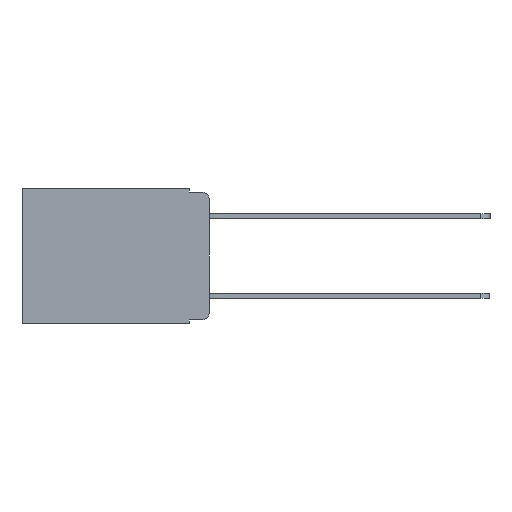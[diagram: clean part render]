
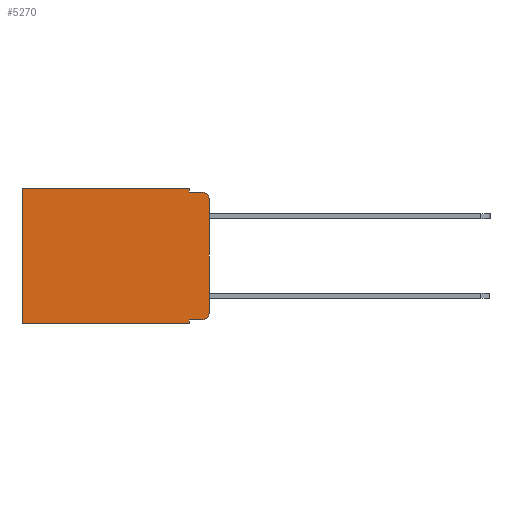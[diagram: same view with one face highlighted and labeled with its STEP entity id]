
A CAD part, left-side view. The second image highlights one B-rep face of the part: STEP entity #5270.
In plain terms, the highlighted planar face has unit normal (-1, 0, 0).
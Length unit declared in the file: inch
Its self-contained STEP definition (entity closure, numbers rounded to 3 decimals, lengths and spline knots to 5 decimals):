
#264 = AXIS2_PLACEMENT_3D ( 'NONE', #13797, #13840, #13702 ) ;
#271 = EDGE_CURVE ( 'NONE', #6532, #20474, #13607, .T. ) ;
#804 = EDGE_LOOP ( 'NONE', ( #8529, #3978, #3660, #8248, #21860, #14214, #15563, #12854, #14196, #1198 ) ) ;
#830 = CARTESIAN_POINT ( 'NONE',  ( 0.298, 0.02, -0.333 ) ) ;
#1198 = ORIENTED_EDGE ( 'NONE', *, *, #18199, .T. ) ;
#1254 = EDGE_CURVE ( 'NONE', #1314, #7741, #17901, .T. ) ;
#1314 = VERTEX_POINT ( 'NONE', #8389 ) ;
#1545 = CARTESIAN_POINT ( 'NONE',  ( 0.298, 0.051, -0.343 ) ) ;
#1615 = AXIS2_PLACEMENT_3D ( 'NONE', #13713, #3214, #15461 ) ;
#1744 = LINE ( 'NONE', #19875, #15191 ) ;
#1932 = CARTESIAN_POINT ( 'NONE',  ( 0.298, 0.02, -0.01 ) ) ;
#1942 = LINE ( 'NONE', #3644, #19841 ) ;
#1971 = DIRECTION ( 'NONE',  ( 0., -1., 0. ) ) ;
#1999 = CARTESIAN_POINT ( 'NONE',  ( 0.298, 0., 0. ) ) ;
#2613 = CARTESIAN_POINT ( 'NONE',  ( 0.298, 0.051, -0.01 ) ) ;
#2896 = DIRECTION ( 'NONE',  ( 0., 0., -1. ) ) ;
#3214 = DIRECTION ( 'NONE',  ( -1., 0., 0. ) ) ;
#3222 = AXIS2_PLACEMENT_3D ( 'NONE', #18643, #19577, #15632 ) ;
#3420 = CARTESIAN_POINT ( 'NONE',  ( 0.298, 0.051, -0.333 ) ) ;
#3644 = CARTESIAN_POINT ( 'NONE',  ( 0.298, 0.051, -0.333 ) ) ;
#3660 = ORIENTED_EDGE ( 'NONE', *, *, #10953, .F. ) ;
#3708 = VECTOR ( 'NONE', #16063, 39.37008 ) ;
#3776 = VECTOR ( 'NONE', #20328, 39.37008 ) ;
#3978 = ORIENTED_EDGE ( 'NONE', *, *, #1254, .T. ) ;
#4663 = EDGE_CURVE ( 'NONE', #6532, #14471, #1744, .T. ) ;
#5270 = ADVANCED_FACE ( 'NONE', ( #14062 ), #10724, .F. ) ;
#6138 = CARTESIAN_POINT ( 'NONE',  ( 0.298, 0.051, -0.01 ) ) ;
#6429 = CARTESIAN_POINT ( 'NONE',  ( 0.298, 0., -0.343 ) ) ;
#6532 = VERTEX_POINT ( 'NONE', #16132 ) ;
#7310 = DIRECTION ( 'NONE',  ( 0., 0., -1. ) ) ;
#7674 = LINE ( 'NONE', #17781, #20296 ) ;
#7741 = VERTEX_POINT ( 'NONE', #1932 ) ;
#8248 = ORIENTED_EDGE ( 'NONE', *, *, #4663, .F. ) ;
#8389 = CARTESIAN_POINT ( 'NONE',  ( 0.298, 0., -0.03 ) ) ;
#8529 = ORIENTED_EDGE ( 'NONE', *, *, #19657, .F. ) ;
#8639 = VECTOR ( 'NONE', #7310, 39.37008 ) ;
#8754 = EDGE_CURVE ( 'NONE', #10099, #18888, #19364, .T. ) ;
#9348 = VERTEX_POINT ( 'NONE', #11978 ) ;
#10099 = VERTEX_POINT ( 'NONE', #3420 ) ;
#10206 = VECTOR ( 'NONE', #2896, 39.37008 ) ;
#10724 = PLANE ( 'NONE',  #3222 ) ;
#10953 = EDGE_CURVE ( 'NONE', #14471, #7741, #20298, .T. ) ;
#11147 = EDGE_CURVE ( 'NONE', #18888, #13577, #17702, .T. ) ;
#11563 = CARTESIAN_POINT ( 'NONE',  ( 0.298, 0.473, 0. ) ) ;
#11771 = VECTOR ( 'NONE', #18257, 39.37008 ) ;
#11978 = CARTESIAN_POINT ( 'NONE',  ( 0.298, 0., -0.313 ) ) ;
#12236 = DIRECTION ( 'NONE',  ( 0., 0., -1. ) ) ;
#12854 = ORIENTED_EDGE ( 'NONE', *, *, #8754, .F. ) ;
#13307 = LINE ( 'NONE', #1999, #8639 ) ;
#13577 = VERTEX_POINT ( 'NONE', #17658 ) ;
#13607 = LINE ( 'NONE', #16015, #3708 ) ;
#13702 = DIRECTION ( 'NONE',  ( 0., 0., -1. ) ) ;
#13713 = CARTESIAN_POINT ( 'NONE',  ( 0.298, 0.02, -0.313 ) ) ;
#13797 = CARTESIAN_POINT ( 'NONE',  ( 0.298, 0.02, -0.03 ) ) ;
#13840 = DIRECTION ( 'NONE',  ( -1., 0., 0. ) ) ;
#14062 = FACE_OUTER_BOUND ( 'NONE', #804, .T. ) ;
#14196 = ORIENTED_EDGE ( 'NONE', *, *, #16644, .T. ) ;
#14214 = ORIENTED_EDGE ( 'NONE', *, *, #17936, .T. ) ;
#14471 = VERTEX_POINT ( 'NONE', #2613 ) ;
#15043 = VERTEX_POINT ( 'NONE', #830 ) ;
#15191 = VECTOR ( 'NONE', #12236, 39.37008 ) ;
#15461 = DIRECTION ( 'NONE',  ( 0., 0., -1. ) ) ;
#15563 = ORIENTED_EDGE ( 'NONE', *, *, #11147, .F. ) ;
#15632 = DIRECTION ( 'NONE',  ( 0., 0., -1. ) ) ;
#16015 = CARTESIAN_POINT ( 'NONE',  ( 0.298, 0., 0. ) ) ;
#16063 = DIRECTION ( 'NONE',  ( 0., 1., 0. ) ) ;
#16067 = DIRECTION ( 'NONE',  ( 0., 0., -1. ) ) ;
#16132 = CARTESIAN_POINT ( 'NONE',  ( 0.298, 0.051, 0. ) ) ;
#16644 = EDGE_CURVE ( 'NONE', #10099, #15043, #1942, .T. ) ;
#17658 = CARTESIAN_POINT ( 'NONE',  ( 0.298, 0.473, -0.343 ) ) ;
#17702 = LINE ( 'NONE', #6429, #3776 ) ;
#17781 = CARTESIAN_POINT ( 'NONE',  ( 0.298, 0.473, 0. ) ) ;
#17901 = CIRCLE ( 'NONE', #264, 0.02 ) ;
#17936 = EDGE_CURVE ( 'NONE', #20474, #13577, #7674, .T. ) ;
#18199 = EDGE_CURVE ( 'NONE', #15043, #9348, #19497, .T. ) ;
#18257 = DIRECTION ( 'NONE',  ( 0., -1., 0. ) ) ;
#18643 = CARTESIAN_POINT ( 'NONE',  ( 0.298, 0., 0. ) ) ;
#18888 = VERTEX_POINT ( 'NONE', #1545 ) ;
#19364 = LINE ( 'NONE', #20137, #10206 ) ;
#19497 = CIRCLE ( 'NONE', #1615, 0.02 ) ;
#19577 = DIRECTION ( 'NONE',  ( 1., 0., 0. ) ) ;
#19657 = EDGE_CURVE ( 'NONE', #1314, #9348, #13307, .T. ) ;
#19841 = VECTOR ( 'NONE', #1971, 39.37008 ) ;
#19875 = CARTESIAN_POINT ( 'NONE',  ( 0.298, 0.051, 0. ) ) ;
#20137 = CARTESIAN_POINT ( 'NONE',  ( 0.298, 0.051, 0. ) ) ;
#20296 = VECTOR ( 'NONE', #16067, 39.37008 ) ;
#20298 = LINE ( 'NONE', #6138, #11771 ) ;
#20328 = DIRECTION ( 'NONE',  ( 0., 1., 0. ) ) ;
#20474 = VERTEX_POINT ( 'NONE', #11563 ) ;
#21860 = ORIENTED_EDGE ( 'NONE', *, *, #271, .T. ) ;
